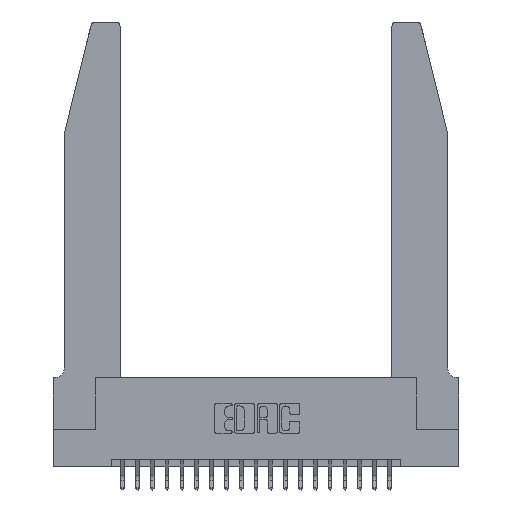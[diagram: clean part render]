
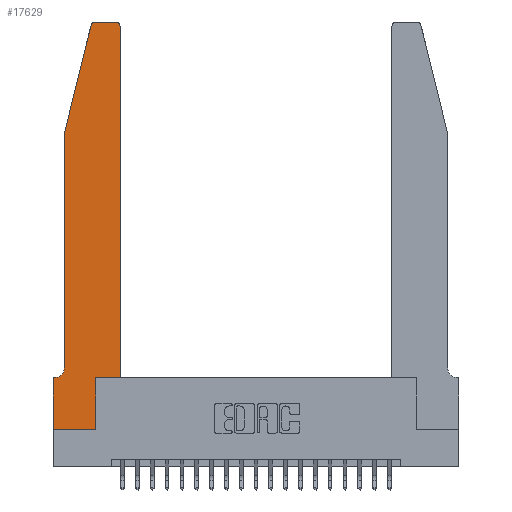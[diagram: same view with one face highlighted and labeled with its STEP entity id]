
A CAD part, top view. The second image highlights one B-rep face of the part: STEP entity #17629.
In plain terms, the highlighted planar face has unit normal (0, 0, 1).
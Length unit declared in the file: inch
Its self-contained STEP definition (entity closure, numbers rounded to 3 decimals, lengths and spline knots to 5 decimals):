
#37 = EDGE_CURVE ( 'NONE', #15803, #8988, #4148, .T. ) ;
#610 = CARTESIAN_POINT ( 'NONE',  ( 0.2865, 0.35, 0.37 ) ) ;
#782 = VERTEX_POINT ( 'NONE', #6431 ) ;
#1013 = DIRECTION ( 'NONE',  ( 0., -1., 0. ) ) ;
#1278 = DIRECTION ( 'NONE',  ( 0., 0., 1. ) ) ;
#1319 = VECTOR ( 'NONE', #9002, 39.37008 ) ;
#1335 = DIRECTION ( 'NONE',  ( 0., 0., 1. ) ) ;
#1422 = EDGE_CURVE ( 'NONE', #9820, #782, #3235, .T. ) ;
#1898 = LINE ( 'NONE', #7185, #1319 ) ;
#2127 = CIRCLE ( 'NONE', #14963, 0.03 ) ;
#2144 = CARTESIAN_POINT ( 'NONE',  ( 0.0055, 0.42, 0.37 ) ) ;
#2567 = CIRCLE ( 'NONE', #9804, 0.03 ) ;
#2770 = CARTESIAN_POINT ( 'NONE',  ( 0.25487, 2.72718, 0.37 ) ) ;
#2793 = EDGE_CURVE ( 'NONE', #2885, #15007, #21993, .T. ) ;
#2885 = VERTEX_POINT ( 'NONE', #2770 ) ;
#2977 = DIRECTION ( 'NONE',  ( 0., 0., 1. ) ) ;
#3046 = VERTEX_POINT ( 'NONE', #20084 ) ;
#3106 = CARTESIAN_POINT ( 'NONE',  ( 0., 0.35, 0.37 ) ) ;
#3166 = VECTOR ( 'NONE', #10733, 39.37008 ) ;
#3235 = LINE ( 'NONE', #13855, #11685 ) ;
#3386 = EDGE_CURVE ( 'NONE', #782, #2885, #2567, .T. ) ;
#3701 = EDGE_CURVE ( 'NONE', #14193, #5791, #18416, .T. ) ;
#3984 = DIRECTION ( 'NONE',  ( -1., 0., 0. ) ) ;
#4148 = LINE ( 'NONE', #10849, #13134 ) ;
#4233 = CARTESIAN_POINT ( 'NONE',  ( 0., 0.35, 0.37 ) ) ;
#4500 = VECTOR ( 'NONE', #15388, 39.37008 ) ;
#4812 = EDGE_LOOP ( 'NONE', ( #6522, #17969, #21976, #16366, #15055, #9032, #15674, #9451, #16139, #18762, #12639, #15958 ) ) ;
#5045 = LINE ( 'NONE', #13726, #4500 ) ;
#5131 = VECTOR ( 'NONE', #5930, 39.37008 ) ;
#5524 = DIRECTION ( 'NONE',  ( 1., 0., 0. ) ) ;
#5791 = VERTEX_POINT ( 'NONE', #610 ) ;
#5930 = DIRECTION ( 'NONE',  ( 1., 0., 0. ) ) ;
#6323 = FACE_OUTER_BOUND ( 'NONE', #4812, .T. ) ;
#6431 = CARTESIAN_POINT ( 'NONE',  ( 0.284, 2.75, 0.37 ) ) ;
#6522 = ORIENTED_EDGE ( 'NONE', *, *, #1422, .T. ) ;
#6777 = VECTOR ( 'NONE', #21112, 39.37008 ) ;
#7185 = CARTESIAN_POINT ( 'NONE',  ( 0.4505, 0.35, 0.37 ) ) ;
#7681 = CARTESIAN_POINT ( 'NONE',  ( 0.2865, 0.35, 0.37 ) ) ;
#8330 = CARTESIAN_POINT ( 'NONE',  ( 0.284, 2.72, 0.37 ) ) ;
#8373 = DIRECTION ( 'NONE',  ( -1., 0., 0. ) ) ;
#8436 = CARTESIAN_POINT ( 'NONE',  ( 0.0755, 0.42, 0.37 ) ) ;
#8629 = VERTEX_POINT ( 'NONE', #12372 ) ;
#8988 = VERTEX_POINT ( 'NONE', #13746 ) ;
#9002 = DIRECTION ( 'NONE',  ( 0., 1., 0. ) ) ;
#9032 = ORIENTED_EDGE ( 'NONE', *, *, #18311, .T. ) ;
#9451 = ORIENTED_EDGE ( 'NONE', *, *, #20191, .T. ) ;
#9545 = CARTESIAN_POINT ( 'NONE',  ( 0.2865, 0., 0.37 ) ) ;
#9804 = AXIS2_PLACEMENT_3D ( 'NONE', #8330, #1278, #5524 ) ;
#9820 = VERTEX_POINT ( 'NONE', #17013 ) ;
#9921 = LINE ( 'NONE', #18249, #5131 ) ;
#10566 = VECTOR ( 'NONE', #8373, 39.37008 ) ;
#10733 = DIRECTION ( 'NONE',  ( -0.239, -0.971, 0. ) ) ;
#10821 = EDGE_CURVE ( 'NONE', #12492, #21519, #17527, .T. ) ;
#10849 = CARTESIAN_POINT ( 'NONE',  ( 0., 0., 0.37 ) ) ;
#10855 = CARTESIAN_POINT ( 'NONE',  ( 0.0755, 2., 0.37 ) ) ;
#11052 = AXIS2_PLACEMENT_3D ( 'NONE', #3106, #1335, #13926 ) ;
#11302 = DIRECTION ( 'NONE',  ( 0., 1., 0. ) ) ;
#11352 = CARTESIAN_POINT ( 'NONE',  ( 0.0755, 2., 0.37 ) ) ;
#11594 = LINE ( 'NONE', #14137, #6777 ) ;
#11685 = VECTOR ( 'NONE', #13801, 39.37008 ) ;
#12372 = CARTESIAN_POINT ( 'NONE',  ( 0.4505, 0.35, 0.37 ) ) ;
#12492 = VERTEX_POINT ( 'NONE', #8436 ) ;
#12639 = ORIENTED_EDGE ( 'NONE', *, *, #22046, .T. ) ;
#13033 = CARTESIAN_POINT ( 'NONE',  ( 0.0055, 0.35, 0.37 ) ) ;
#13134 = VECTOR ( 'NONE', #1013, 39.37008 ) ;
#13156 = EDGE_CURVE ( 'NONE', #15007, #12492, #5045, .T. ) ;
#13726 = CARTESIAN_POINT ( 'NONE',  ( 0.0755, 2., 0.37 ) ) ;
#13733 = CARTESIAN_POINT ( 'NONE',  ( 0.4205, 2.72, 0.37 ) ) ;
#13746 = CARTESIAN_POINT ( 'NONE',  ( 0., 0., 0.37 ) ) ;
#13794 = VECTOR ( 'NONE', #11302, 39.37008 ) ;
#13801 = DIRECTION ( 'NONE',  ( -1., 0., 0. ) ) ;
#13855 = CARTESIAN_POINT ( 'NONE',  ( 0.2605, 2.75, 0.37 ) ) ;
#13926 = DIRECTION ( 'NONE',  ( 1., 0., 0. ) ) ;
#14137 = CARTESIAN_POINT ( 'NONE',  ( 0., 0., 0.37 ) ) ;
#14193 = VERTEX_POINT ( 'NONE', #9545 ) ;
#14695 = DIRECTION ( 'NONE',  ( 0., 0., -1. ) ) ;
#14963 = AXIS2_PLACEMENT_3D ( 'NONE', #13733, #2977, #15473 ) ;
#15007 = VERTEX_POINT ( 'NONE', #10855 ) ;
#15055 = ORIENTED_EDGE ( 'NONE', *, *, #10821, .T. ) ;
#15388 = DIRECTION ( 'NONE',  ( 0., -1., 0. ) ) ;
#15473 = DIRECTION ( 'NONE',  ( 1., 0., 0. ) ) ;
#15674 = ORIENTED_EDGE ( 'NONE', *, *, #37, .T. ) ;
#15779 = LINE ( 'NONE', #22347, #10566 ) ;
#15803 = VERTEX_POINT ( 'NONE', #4233 ) ;
#15958 = ORIENTED_EDGE ( 'NONE', *, *, #22988, .T. ) ;
#16139 = ORIENTED_EDGE ( 'NONE', *, *, #3701, .T. ) ;
#16366 = ORIENTED_EDGE ( 'NONE', *, *, #13156, .T. ) ;
#17013 = CARTESIAN_POINT ( 'NONE',  ( 0.4205, 2.75, 0.37 ) ) ;
#17527 = CIRCLE ( 'NONE', #19894, 0.07 ) ;
#17629 = ADVANCED_FACE ( 'NONE', ( #6323 ), #22573, .T. ) ;
#17969 = ORIENTED_EDGE ( 'NONE', *, *, #3386, .T. ) ;
#18249 = CARTESIAN_POINT ( 'NONE',  ( 0.4505, 0.35, 0.37 ) ) ;
#18311 = EDGE_CURVE ( 'NONE', #21519, #15803, #15779, .T. ) ;
#18416 = LINE ( 'NONE', #7681, #13794 ) ;
#18762 = ORIENTED_EDGE ( 'NONE', *, *, #19786, .T. ) ;
#19786 = EDGE_CURVE ( 'NONE', #5791, #8629, #9921, .T. ) ;
#19894 = AXIS2_PLACEMENT_3D ( 'NONE', #2144, #14695, #3984 ) ;
#20084 = CARTESIAN_POINT ( 'NONE',  ( 0.4505, 2.72, 0.37 ) ) ;
#20191 = EDGE_CURVE ( 'NONE', #8988, #14193, #11594, .T. ) ;
#21112 = DIRECTION ( 'NONE',  ( 1., 0., 0. ) ) ;
#21519 = VERTEX_POINT ( 'NONE', #13033 ) ;
#21976 = ORIENTED_EDGE ( 'NONE', *, *, #2793, .T. ) ;
#21993 = LINE ( 'NONE', #11352, #3166 ) ;
#22046 = EDGE_CURVE ( 'NONE', #8629, #3046, #1898, .T. ) ;
#22347 = CARTESIAN_POINT ( 'NONE',  ( 0.0755, 0.35, 0.37 ) ) ;
#22573 = PLANE ( 'NONE',  #11052 ) ;
#22988 = EDGE_CURVE ( 'NONE', #3046, #9820, #2127, .T. ) ;
